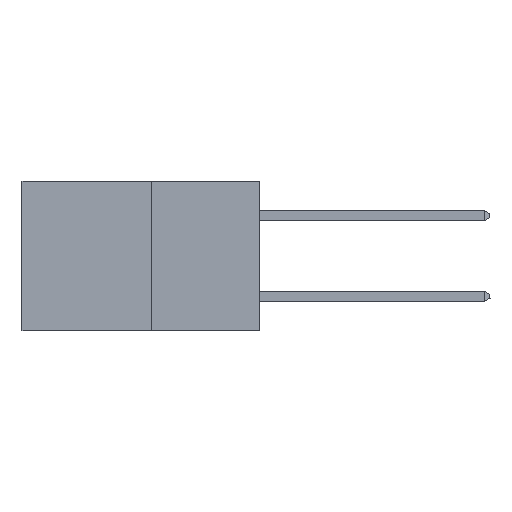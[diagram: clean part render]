
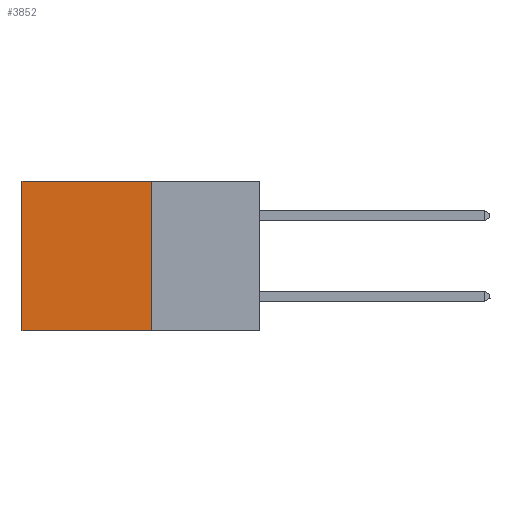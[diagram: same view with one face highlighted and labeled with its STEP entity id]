
A CAD part, left-side view. The second image highlights one B-rep face of the part: STEP entity #3852.
In plain terms, the highlighted planar face has unit normal (-1, 0, 0).
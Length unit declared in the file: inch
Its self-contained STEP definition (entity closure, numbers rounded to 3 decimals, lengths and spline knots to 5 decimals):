
#117 = CARTESIAN_POINT ( 'NONE',  ( 0.277, 0.27, -0.37 ) ) ;
#170 = DIRECTION ( 'NONE',  ( 1., 0., 0. ) ) ;
#200 = PLANE ( 'NONE',  #1052 ) ;
#340 = ORIENTED_EDGE ( 'NONE', *, *, #1684, .F. ) ;
#1052 = AXIS2_PLACEMENT_3D ( 'NONE', #117, #170, #2292 ) ;
#1219 = CARTESIAN_POINT ( 'NONE',  ( 0.277, 0.27, -0.37 ) ) ;
#1265 = VERTEX_POINT ( 'NONE', #10425 ) ;
#1329 = CARTESIAN_POINT ( 'NONE',  ( 0.277, 0.59, 0. ) ) ;
#1471 = VERTEX_POINT ( 'NONE', #10638 ) ;
#1684 = EDGE_CURVE ( 'NONE', #1471, #1265, #6627, .T. ) ;
#2292 = DIRECTION ( 'NONE',  ( 0., 0., -1. ) ) ;
#2712 = LINE ( 'NONE', #10725, #5836 ) ;
#2727 = VECTOR ( 'NONE', #3124, 39.37008 ) ;
#3121 = EDGE_CURVE ( 'NONE', #6799, #1265, #9035, .T. ) ;
#3124 = DIRECTION ( 'NONE',  ( 0., 0., -1. ) ) ;
#3852 = ADVANCED_FACE ( 'NONE', ( #14337 ), #200, .F. ) ;
#4748 = DIRECTION ( 'NONE',  ( 0., 1., 0. ) ) ;
#5115 = CARTESIAN_POINT ( 'NONE',  ( 0.277, 0.59, -0.37 ) ) ;
#5616 = EDGE_CURVE ( 'NONE', #6278, #1471, #9507, .T. ) ;
#5836 = VECTOR ( 'NONE', #4748, 39.37008 ) ;
#5944 = VECTOR ( 'NONE', #10882, 39.37008 ) ;
#6234 = ORIENTED_EDGE ( 'NONE', *, *, #3121, .T. ) ;
#6278 = VERTEX_POINT ( 'NONE', #7832 ) ;
#6627 = LINE ( 'NONE', #1219, #7002 ) ;
#6799 = VERTEX_POINT ( 'NONE', #1329 ) ;
#7002 = VECTOR ( 'NONE', #14807, 39.37008 ) ;
#7832 = CARTESIAN_POINT ( 'NONE',  ( 0.277, 0.27, 0. ) ) ;
#8331 = EDGE_LOOP ( 'NONE', ( #6234, #340, #10174, #10550 ) ) ;
#9035 = LINE ( 'NONE', #5115, #2727 ) ;
#9507 = LINE ( 'NONE', #10860, #5944 ) ;
#10174 = ORIENTED_EDGE ( 'NONE', *, *, #5616, .F. ) ;
#10425 = CARTESIAN_POINT ( 'NONE',  ( 0.277, 0.59, -0.37 ) ) ;
#10550 = ORIENTED_EDGE ( 'NONE', *, *, #12487, .T. ) ;
#10638 = CARTESIAN_POINT ( 'NONE',  ( 0.277, 0.27, -0.37 ) ) ;
#10725 = CARTESIAN_POINT ( 'NONE',  ( 0.277, 0.27, 0. ) ) ;
#10860 = CARTESIAN_POINT ( 'NONE',  ( 0.277, 0.27, -0.37 ) ) ;
#10882 = DIRECTION ( 'NONE',  ( 0., 0., -1. ) ) ;
#12487 = EDGE_CURVE ( 'NONE', #6278, #6799, #2712, .T. ) ;
#14337 = FACE_OUTER_BOUND ( 'NONE', #8331, .T. ) ;
#14807 = DIRECTION ( 'NONE',  ( 0., 1., 0. ) ) ;
